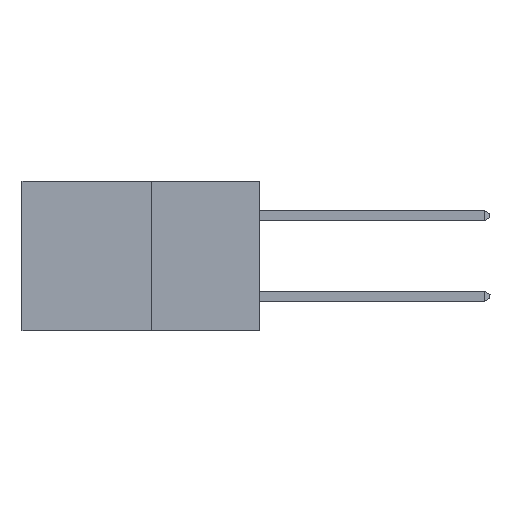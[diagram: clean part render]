
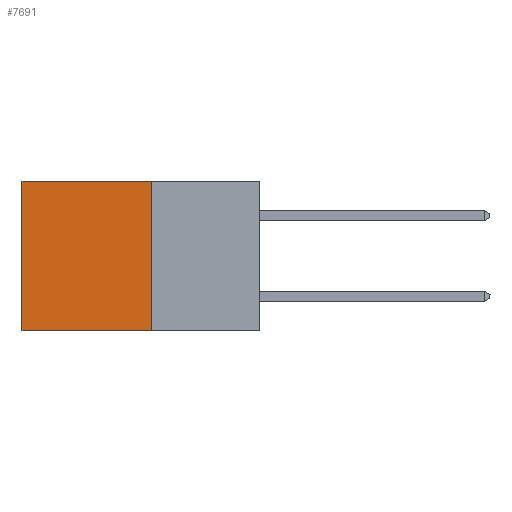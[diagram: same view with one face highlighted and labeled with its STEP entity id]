
A CAD part, left-side view. The second image highlights one B-rep face of the part: STEP entity #7691.
In plain terms, the highlighted planar face has unit normal (-1, 0, 0).
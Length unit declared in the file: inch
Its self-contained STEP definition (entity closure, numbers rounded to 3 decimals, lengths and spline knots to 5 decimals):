
#689 = VECTOR ( 'NONE', #6132, 39.37008 ) ;
#1091 = AXIS2_PLACEMENT_3D ( 'NONE', #1400, #5149, #2916 ) ;
#1400 = CARTESIAN_POINT ( 'NONE',  ( 0.277, 0.27, -0.37 ) ) ;
#1749 = ORIENTED_EDGE ( 'NONE', *, *, #6870, .F. ) ;
#1996 = ORIENTED_EDGE ( 'NONE', *, *, #6311, .T. ) ;
#2001 = CARTESIAN_POINT ( 'NONE',  ( 0.277, 0.59, -0.37 ) ) ;
#2159 = PLANE ( 'NONE',  #1091 ) ;
#2697 = LINE ( 'NONE', #5756, #689 ) ;
#2716 = CARTESIAN_POINT ( 'NONE',  ( 0.277, 0.27, -0.37 ) ) ;
#2916 = DIRECTION ( 'NONE',  ( 0., 0., -1. ) ) ;
#2991 = DIRECTION ( 'NONE',  ( 0., 1., 0. ) ) ;
#3003 = VECTOR ( 'NONE', #2991, 39.37008 ) ;
#3697 = VERTEX_POINT ( 'NONE', #2001 ) ;
#3739 = ORIENTED_EDGE ( 'NONE', *, *, #4358, .F. ) ;
#3770 = VERTEX_POINT ( 'NONE', #2716 ) ;
#3949 = CARTESIAN_POINT ( 'NONE',  ( 0.277, 0.27, -0.37 ) ) ;
#4358 = EDGE_CURVE ( 'NONE', #4929, #3770, #5631, .T. ) ;
#4867 = FACE_OUTER_BOUND ( 'NONE', #5292, .T. ) ;
#4929 = VERTEX_POINT ( 'NONE', #6415 ) ;
#5149 = DIRECTION ( 'NONE',  ( 1., 0., 0. ) ) ;
#5231 = CARTESIAN_POINT ( 'NONE',  ( 0.277, 0.27, -0.37 ) ) ;
#5292 = EDGE_LOOP ( 'NONE', ( #7520, #1749, #3739, #1996 ) ) ;
#5631 = LINE ( 'NONE', #3949, #9027 ) ;
#5750 = DIRECTION ( 'NONE',  ( 0., 0., -1. ) ) ;
#5756 = CARTESIAN_POINT ( 'NONE',  ( 0.277, 0.27, 0. ) ) ;
#6132 = DIRECTION ( 'NONE',  ( 0., 1., 0. ) ) ;
#6267 = EDGE_CURVE ( 'NONE', #8581, #3697, #8093, .T. ) ;
#6311 = EDGE_CURVE ( 'NONE', #4929, #8581, #2697, .T. ) ;
#6415 = CARTESIAN_POINT ( 'NONE',  ( 0.277, 0.27, 0. ) ) ;
#6870 = EDGE_CURVE ( 'NONE', #3770, #3697, #7263, .T. ) ;
#7263 = LINE ( 'NONE', #5231, #3003 ) ;
#7340 = CARTESIAN_POINT ( 'NONE',  ( 0.277, 0.59, -0.37 ) ) ;
#7520 = ORIENTED_EDGE ( 'NONE', *, *, #6267, .T. ) ;
#7542 = DIRECTION ( 'NONE',  ( 0., 0., -1. ) ) ;
#7639 = CARTESIAN_POINT ( 'NONE',  ( 0.277, 0.59, 0. ) ) ;
#7691 = ADVANCED_FACE ( 'NONE', ( #4867 ), #2159, .F. ) ;
#7876 = VECTOR ( 'NONE', #7542, 39.37008 ) ;
#8093 = LINE ( 'NONE', #7340, #7876 ) ;
#8581 = VERTEX_POINT ( 'NONE', #7639 ) ;
#9027 = VECTOR ( 'NONE', #5750, 39.37008 ) ;
